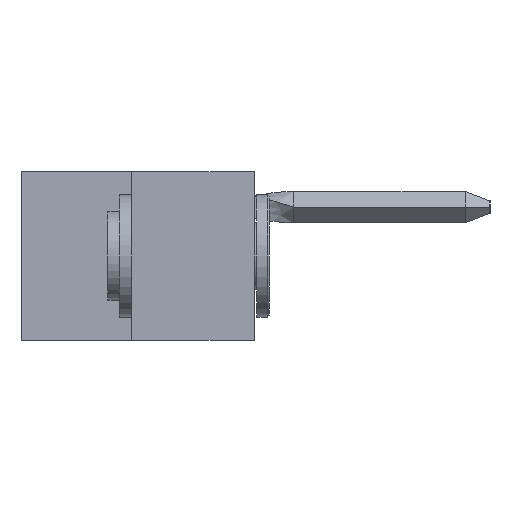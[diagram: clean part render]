
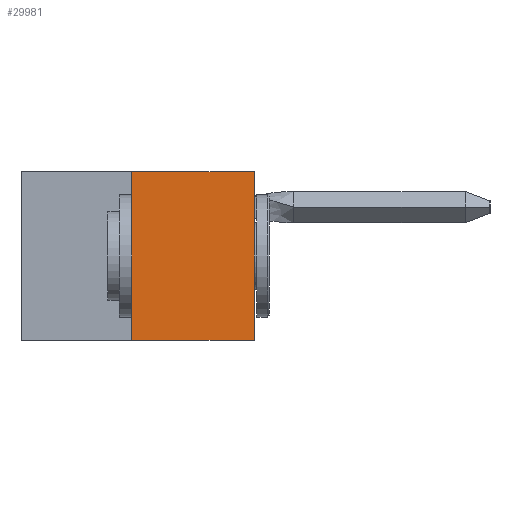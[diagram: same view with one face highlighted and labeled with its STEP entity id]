
A CAD part, left-side view. The second image highlights one B-rep face of the part: STEP entity #29981.
In plain terms, the highlighted planar face has unit normal (-1, 0, 0).
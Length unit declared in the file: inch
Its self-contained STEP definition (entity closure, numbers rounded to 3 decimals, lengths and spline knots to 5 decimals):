
#92 = DIRECTION ( 'NONE',  ( 0., 0., -1. ) ) ;
#410 = VECTOR ( 'NONE', #6914, 39.37008 ) ;
#1447 = CARTESIAN_POINT ( 'NONE',  ( 0., 0., 0. ) ) ;
#2111 = VECTOR ( 'NONE', #18486, 39.37008 ) ;
#2932 = LINE ( 'NONE', #20764, #28922 ) ;
#5086 = VERTEX_POINT ( 'NONE', #13961 ) ;
#6914 = DIRECTION ( 'NONE',  ( 0., 0., 1. ) ) ;
#8917 = DIRECTION ( 'NONE',  ( 0., 0., 1. ) ) ;
#9040 = EDGE_CURVE ( 'NONE', #12159, #5086, #2932, .T. ) ;
#10122 = PLANE ( 'NONE',  #18110 ) ;
#10374 = ORIENTED_EDGE ( 'NONE', *, *, #30204, .F. ) ;
#11033 = VERTEX_POINT ( 'NONE', #20007 ) ;
#11048 = LINE ( 'NONE', #14292, #410 ) ;
#12159 = VERTEX_POINT ( 'NONE', #14763 ) ;
#12651 = CARTESIAN_POINT ( 'NONE',  ( 0., 0.473, 0. ) ) ;
#13961 = CARTESIAN_POINT ( 'NONE',  ( 0., 0., -0.343 ) ) ;
#13966 = CARTESIAN_POINT ( 'NONE',  ( 0., 0.25, 0. ) ) ;
#14292 = CARTESIAN_POINT ( 'NONE',  ( 0., 0.25, 0. ) ) ;
#14763 = CARTESIAN_POINT ( 'NONE',  ( 0., 0.25, -0.343 ) ) ;
#16267 = LINE ( 'NONE', #28351, #2111 ) ;
#18110 = AXIS2_PLACEMENT_3D ( 'NONE', #12651, #27749, #92 ) ;
#18486 = DIRECTION ( 'NONE',  ( 0., -1., 0. ) ) ;
#20007 = CARTESIAN_POINT ( 'NONE',  ( 0., 0., 0. ) ) ;
#20022 = ORIENTED_EDGE ( 'NONE', *, *, #28107, .F. ) ;
#20764 = CARTESIAN_POINT ( 'NONE',  ( 0., 0.473, -0.343 ) ) ;
#22359 = EDGE_CURVE ( 'NONE', #5086, #11033, #31558, .T. ) ;
#22725 = ORIENTED_EDGE ( 'NONE', *, *, #9040, .T. ) ;
#23627 = DIRECTION ( 'NONE',  ( 0., -1., 0. ) ) ;
#24898 = VERTEX_POINT ( 'NONE', #13966 ) ;
#27255 = FACE_OUTER_BOUND ( 'NONE', #30574, .T. ) ;
#27749 = DIRECTION ( 'NONE',  ( 1., 0., 0. ) ) ;
#28107 = EDGE_CURVE ( 'NONE', #24898, #11033, #16267, .T. ) ;
#28351 = CARTESIAN_POINT ( 'NONE',  ( 0., 0.473, 0. ) ) ;
#28790 = VECTOR ( 'NONE', #8917, 39.37008 ) ;
#28922 = VECTOR ( 'NONE', #23627, 39.37008 ) ;
#29981 = ADVANCED_FACE ( 'NONE', ( #27255 ), #10122, .F. ) ;
#30204 = EDGE_CURVE ( 'NONE', #12159, #24898, #11048, .T. ) ;
#30574 = EDGE_LOOP ( 'NONE', ( #20022, #10374, #22725, #30961 ) ) ;
#30961 = ORIENTED_EDGE ( 'NONE', *, *, #22359, .T. ) ;
#31558 = LINE ( 'NONE', #1447, #28790 ) ;
